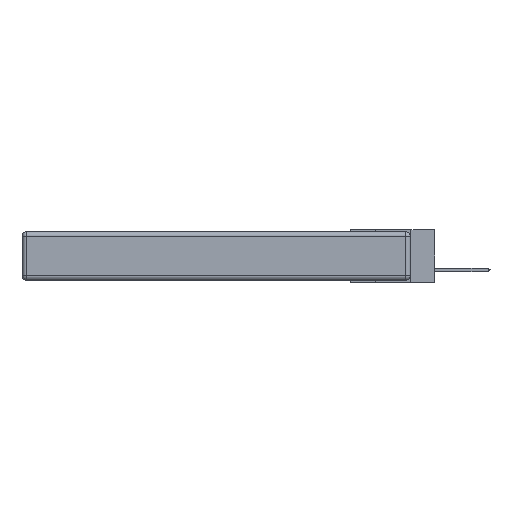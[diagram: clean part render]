
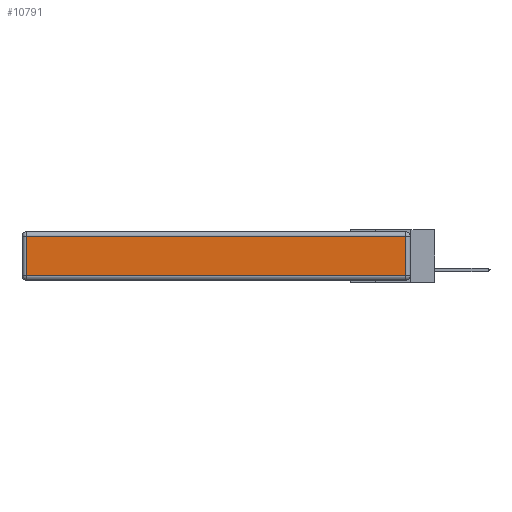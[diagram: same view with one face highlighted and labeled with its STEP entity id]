
A CAD part, left-side view. The second image highlights one B-rep face of the part: STEP entity #10791.
In plain terms, the highlighted planar face has unit normal (-1, 0, 0).
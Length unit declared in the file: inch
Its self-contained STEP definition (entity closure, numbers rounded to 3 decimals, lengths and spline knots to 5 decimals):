
#308 = VECTOR ( 'NONE', #21739, 39.37008 ) ;
#1507 = FACE_OUTER_BOUND ( 'NONE', #24403, .T. ) ;
#1904 = ORIENTED_EDGE ( 'NONE', *, *, #20727, .T. ) ;
#3094 = VERTEX_POINT ( 'NONE', #3503 ) ;
#3328 = CARTESIAN_POINT ( 'NONE',  ( 0., 0., -0.313 ) ) ;
#3503 = CARTESIAN_POINT ( 'NONE',  ( 0., 0.03, -0.313 ) ) ;
#3643 = DIRECTION ( 'NONE',  ( 0., 0., -1. ) ) ;
#4063 = LINE ( 'NONE', #3328, #308 ) ;
#5480 = ORIENTED_EDGE ( 'NONE', *, *, #29859, .T. ) ;
#5498 = CARTESIAN_POINT ( 'NONE',  ( 0., 2.75, -0.03 ) ) ;
#5545 = CARTESIAN_POINT ( 'NONE',  ( 0., 2.72, -0.313 ) ) ;
#5601 = VERTEX_POINT ( 'NONE', #5545 ) ;
#8355 = LINE ( 'NONE', #13796, #26896 ) ;
#9060 = VECTOR ( 'NONE', #3643, 39.37008 ) ;
#9409 = CARTESIAN_POINT ( 'NONE',  ( 0., 2.72, -0.03 ) ) ;
#10791 = ADVANCED_FACE ( 'NONE', ( #1507 ), #28020, .T. ) ;
#11647 = CARTESIAN_POINT ( 'NONE',  ( 0., 2.72, -0.343 ) ) ;
#12209 = CARTESIAN_POINT ( 'NONE',  ( 0., 0., -0.343 ) ) ;
#12814 = VERTEX_POINT ( 'NONE', #9409 ) ;
#13796 = CARTESIAN_POINT ( 'NONE',  ( 0., 0.03, -0.343 ) ) ;
#14323 = CARTESIAN_POINT ( 'NONE',  ( 0., 0.03, -0.03 ) ) ;
#14760 = LINE ( 'NONE', #5498, #22165 ) ;
#16055 = LINE ( 'NONE', #11647, #9060 ) ;
#17052 = ORIENTED_EDGE ( 'NONE', *, *, #24789, .T. ) ;
#17234 = EDGE_CURVE ( 'NONE', #19151, #12814, #14760, .T. ) ;
#18938 = DIRECTION ( 'NONE',  ( 0., 1., 0. ) ) ;
#19151 = VERTEX_POINT ( 'NONE', #14323 ) ;
#20727 = EDGE_CURVE ( 'NONE', #3094, #19151, #8355, .T. ) ;
#21739 = DIRECTION ( 'NONE',  ( 0., -1., 0. ) ) ;
#22165 = VECTOR ( 'NONE', #18938, 39.37008 ) ;
#24403 = EDGE_LOOP ( 'NONE', ( #17052, #1904, #31949, #5480 ) ) ;
#24789 = EDGE_CURVE ( 'NONE', #5601, #3094, #4063, .T. ) ;
#25793 = AXIS2_PLACEMENT_3D ( 'NONE', #12209, #33286, #25817 ) ;
#25817 = DIRECTION ( 'NONE',  ( 0., 0., 1. ) ) ;
#26896 = VECTOR ( 'NONE', #29488, 39.37008 ) ;
#28020 = PLANE ( 'NONE',  #25793 ) ;
#29488 = DIRECTION ( 'NONE',  ( 0., 0., 1. ) ) ;
#29859 = EDGE_CURVE ( 'NONE', #12814, #5601, #16055, .T. ) ;
#31949 = ORIENTED_EDGE ( 'NONE', *, *, #17234, .T. ) ;
#33286 = DIRECTION ( 'NONE',  ( -1., 0., 0. ) ) ;
